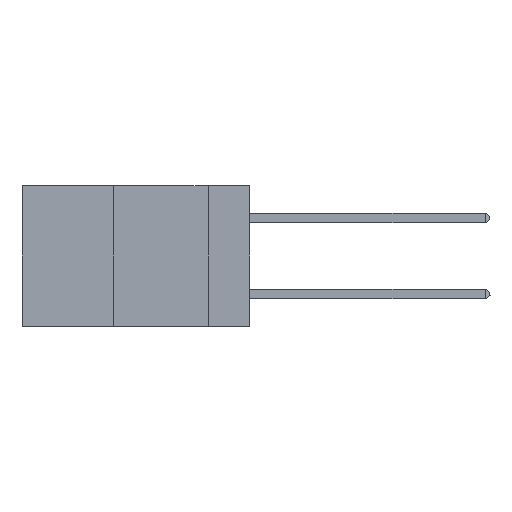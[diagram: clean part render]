
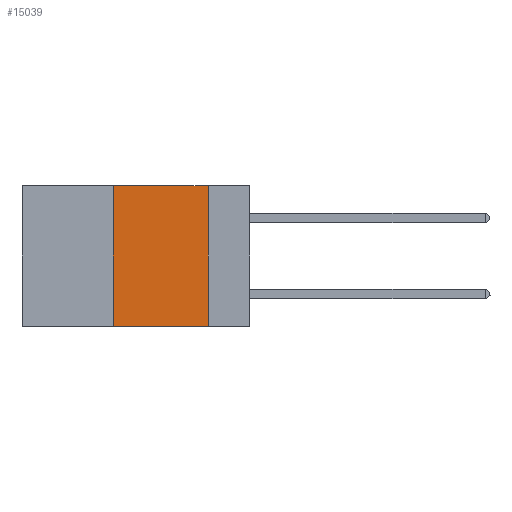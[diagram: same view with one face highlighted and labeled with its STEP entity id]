
A CAD part, left-side view. The second image highlights one B-rep face of the part: STEP entity #15039.
In plain terms, the highlighted planar face has unit normal (-1, 0, 0).
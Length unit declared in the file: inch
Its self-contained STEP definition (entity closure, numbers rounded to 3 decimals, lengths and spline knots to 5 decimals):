
#558 = ORIENTED_EDGE ( 'NONE', *, *, #4096, .F. ) ;
#945 = VECTOR ( 'NONE', #7265, 39.37008 ) ;
#1021 = AXIS2_PLACEMENT_3D ( 'NONE', #13167, #17355, #9321 ) ;
#3044 = PLANE ( 'NONE',  #1021 ) ;
#3294 = VERTEX_POINT ( 'NONE', #19840 ) ;
#3369 = VERTEX_POINT ( 'NONE', #20279 ) ;
#4096 = EDGE_CURVE ( 'NONE', #3369, #10915, #9680, .T. ) ;
#5444 = EDGE_CURVE ( 'NONE', #12802, #3294, #17509, .T. ) ;
#5591 = ORIENTED_EDGE ( 'NONE', *, *, #18122, .F. ) ;
#6520 = ORIENTED_EDGE ( 'NONE', *, *, #5444, .T. ) ;
#6884 = FACE_OUTER_BOUND ( 'NONE', #18979, .T. ) ;
#6943 = LINE ( 'NONE', #12000, #14235 ) ;
#7000 = CARTESIAN_POINT ( 'NONE',  ( 0., 0.36, -0.37 ) ) ;
#7265 = DIRECTION ( 'NONE',  ( 0., -1., 0. ) ) ;
#9136 = CARTESIAN_POINT ( 'NONE',  ( 0., 0.36, 0. ) ) ;
#9321 = DIRECTION ( 'NONE',  ( 0., 0., -1. ) ) ;
#9680 = LINE ( 'NONE', #19326, #945 ) ;
#10208 = VECTOR ( 'NONE', #14847, 39.37008 ) ;
#10915 = VERTEX_POINT ( 'NONE', #22878 ) ;
#12000 = CARTESIAN_POINT ( 'NONE',  ( 0., 0.11, 0. ) ) ;
#12011 = DIRECTION ( 'NONE',  ( 0., 0., -1. ) ) ;
#12802 = VERTEX_POINT ( 'NONE', #7000 ) ;
#13167 = CARTESIAN_POINT ( 'NONE',  ( 0., 0.6, 0. ) ) ;
#13229 = EDGE_CURVE ( 'NONE', #10915, #3294, #6943, .T. ) ;
#14235 = VECTOR ( 'NONE', #12011, 39.37008 ) ;
#14847 = DIRECTION ( 'NONE',  ( 0., -1., 0. ) ) ;
#15019 = CARTESIAN_POINT ( 'NONE',  ( 0., 0.6, -0.37 ) ) ;
#15039 = ADVANCED_FACE ( 'NONE', ( #6884 ), #3044, .F. ) ;
#16507 = VECTOR ( 'NONE', #19025, 39.37008 ) ;
#17355 = DIRECTION ( 'NONE',  ( 1., 0., 0. ) ) ;
#17509 = LINE ( 'NONE', #15019, #10208 ) ;
#18122 = EDGE_CURVE ( 'NONE', #12802, #3369, #25297, .T. ) ;
#18979 = EDGE_LOOP ( 'NONE', ( #25430, #558, #5591, #6520 ) ) ;
#19025 = DIRECTION ( 'NONE',  ( 0., 0., 1. ) ) ;
#19326 = CARTESIAN_POINT ( 'NONE',  ( 0., 0.6, 0. ) ) ;
#19840 = CARTESIAN_POINT ( 'NONE',  ( 0., 0.11, -0.37 ) ) ;
#20279 = CARTESIAN_POINT ( 'NONE',  ( 0., 0.36, 0. ) ) ;
#22878 = CARTESIAN_POINT ( 'NONE',  ( 0., 0.11, 0. ) ) ;
#25297 = LINE ( 'NONE', #9136, #16507 ) ;
#25430 = ORIENTED_EDGE ( 'NONE', *, *, #13229, .F. ) ;
